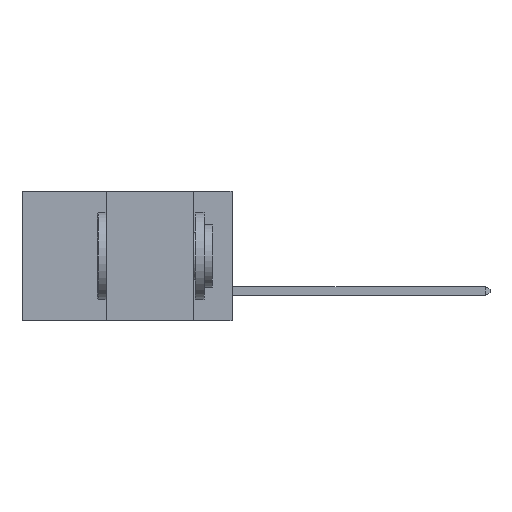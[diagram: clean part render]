
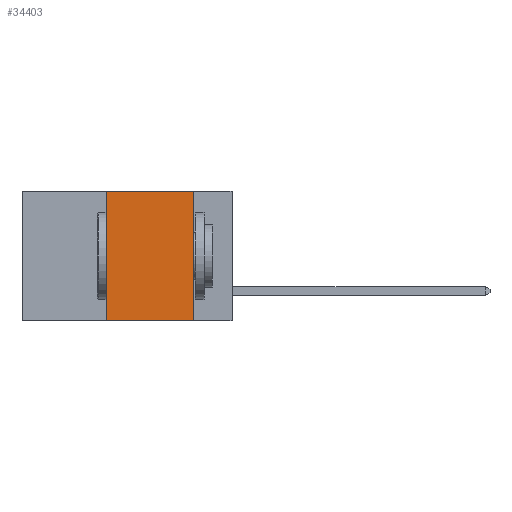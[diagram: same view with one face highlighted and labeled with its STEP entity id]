
A CAD part, left-side view. The second image highlights one B-rep face of the part: STEP entity #34403.
In plain terms, the highlighted planar face has unit normal (-1, 0, 0).
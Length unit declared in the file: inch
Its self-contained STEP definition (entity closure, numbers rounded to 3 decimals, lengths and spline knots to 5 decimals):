
#1995 = CARTESIAN_POINT ( 'NONE',  ( 0., 0.36, 0. ) ) ;
#2632 = ORIENTED_EDGE ( 'NONE', *, *, #34192, .F. ) ;
#3084 = DIRECTION ( 'NONE',  ( 0., -1., 0. ) ) ;
#3776 = VERTEX_POINT ( 'NONE', #28291 ) ;
#4678 = CARTESIAN_POINT ( 'NONE',  ( 0., 0.11, 0. ) ) ;
#7386 = LINE ( 'NONE', #22480, #39986 ) ;
#7516 = EDGE_LOOP ( 'NONE', ( #2632, #10993, #24909, #29825 ) ) ;
#9344 = LINE ( 'NONE', #36028, #10312 ) ;
#10312 = VECTOR ( 'NONE', #29523, 39.37008 ) ;
#10993 = ORIENTED_EDGE ( 'NONE', *, *, #34320, .F. ) ;
#12992 = DIRECTION ( 'NONE',  ( 0., 0., -1. ) ) ;
#13227 = VECTOR ( 'NONE', #17903, 39.37008 ) ;
#13818 = VERTEX_POINT ( 'NONE', #17426 ) ;
#13879 = VECTOR ( 'NONE', #3084, 39.37008 ) ;
#14211 = LINE ( 'NONE', #1995, #13227 ) ;
#17426 = CARTESIAN_POINT ( 'NONE',  ( 0., 0.36, 0. ) ) ;
#17699 = PLANE ( 'NONE',  #34386 ) ;
#17903 = DIRECTION ( 'NONE',  ( 0., 0., 1. ) ) ;
#18821 = CARTESIAN_POINT ( 'NONE',  ( 0., 0.6, -0.37 ) ) ;
#22480 = CARTESIAN_POINT ( 'NONE',  ( 0., 0.11, 0. ) ) ;
#23735 = DIRECTION ( 'NONE',  ( 1., 0., 0. ) ) ;
#23877 = DIRECTION ( 'NONE',  ( 0., 0., -1. ) ) ;
#24682 = CARTESIAN_POINT ( 'NONE',  ( 0., 0.11, -0.37 ) ) ;
#24909 = ORIENTED_EDGE ( 'NONE', *, *, #40725, .F. ) ;
#27142 = FACE_OUTER_BOUND ( 'NONE', #7516, .T. ) ;
#28291 = CARTESIAN_POINT ( 'NONE',  ( 0., 0.36, -0.37 ) ) ;
#29523 = DIRECTION ( 'NONE',  ( 0., -1., 0. ) ) ;
#29825 = ORIENTED_EDGE ( 'NONE', *, *, #33348, .T. ) ;
#30221 = CARTESIAN_POINT ( 'NONE',  ( 0., 0.6, 0. ) ) ;
#30785 = VERTEX_POINT ( 'NONE', #4678 ) ;
#32637 = VERTEX_POINT ( 'NONE', #24682 ) ;
#33348 = EDGE_CURVE ( 'NONE', #3776, #32637, #35091, .T. ) ;
#34192 = EDGE_CURVE ( 'NONE', #30785, #32637, #7386, .T. ) ;
#34320 = EDGE_CURVE ( 'NONE', #13818, #30785, #9344, .T. ) ;
#34386 = AXIS2_PLACEMENT_3D ( 'NONE', #30221, #23735, #23877 ) ;
#34403 = ADVANCED_FACE ( 'NONE', ( #27142 ), #17699, .F. ) ;
#35091 = LINE ( 'NONE', #18821, #13879 ) ;
#36028 = CARTESIAN_POINT ( 'NONE',  ( 0., 0.6, 0. ) ) ;
#39986 = VECTOR ( 'NONE', #12992, 39.37008 ) ;
#40725 = EDGE_CURVE ( 'NONE', #3776, #13818, #14211, .T. ) ;
